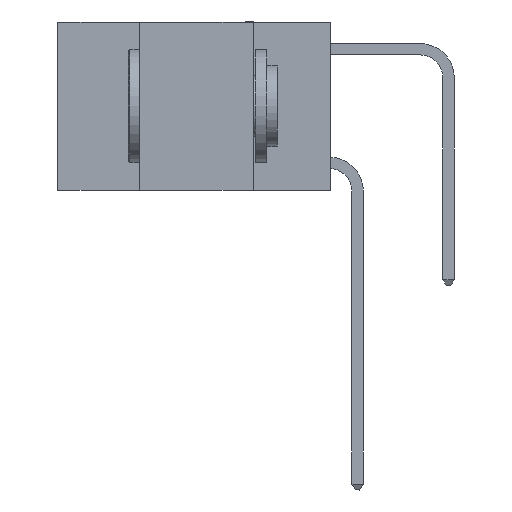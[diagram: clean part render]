
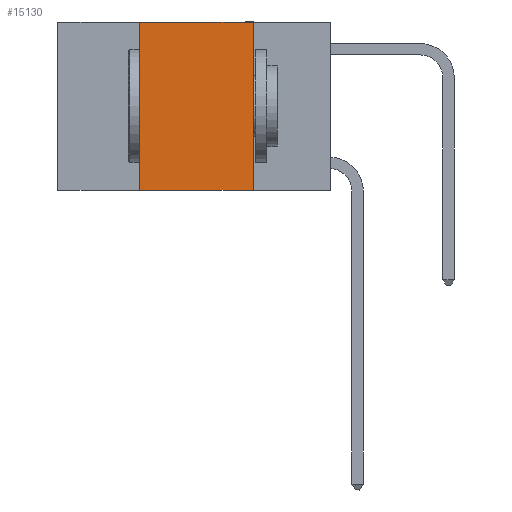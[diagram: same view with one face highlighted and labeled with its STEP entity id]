
A CAD part, left-side view. The second image highlights one B-rep face of the part: STEP entity #15130.
In plain terms, the highlighted planar face has unit normal (-1, 0, 0).
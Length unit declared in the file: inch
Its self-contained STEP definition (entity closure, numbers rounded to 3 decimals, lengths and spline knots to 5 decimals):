
#599 = LINE ( 'NONE', #7512, #14820 ) ;
#1552 = CARTESIAN_POINT ( 'NONE',  ( 0., 0.6, 0. ) ) ;
#2569 = AXIS2_PLACEMENT_3D ( 'NONE', #1552, #24740, #5537 ) ;
#2822 = EDGE_CURVE ( 'NONE', #22975, #13338, #5802, .T. ) ;
#3178 = ORIENTED_EDGE ( 'NONE', *, *, #8623, .F. ) ;
#3203 = ORIENTED_EDGE ( 'NONE', *, *, #2822, .T. ) ;
#3492 = PLANE ( 'NONE',  #2569 ) ;
#4155 = CARTESIAN_POINT ( 'NONE',  ( 0., 0.17, -0.37 ) ) ;
#4890 = DIRECTION ( 'NONE',  ( 0., 0., 1. ) ) ;
#5073 = DIRECTION ( 'NONE',  ( 0., -1., 0. ) ) ;
#5537 = DIRECTION ( 'NONE',  ( 0., 0., -1. ) ) ;
#5802 = LINE ( 'NONE', #12275, #10762 ) ;
#7512 = CARTESIAN_POINT ( 'NONE',  ( 0., 0.17, 0. ) ) ;
#8623 = EDGE_CURVE ( 'NONE', #11925, #20323, #9835, .T. ) ;
#8648 = EDGE_LOOP ( 'NONE', ( #23284, #3178, #22267, #3203 ) ) ;
#9672 = FACE_OUTER_BOUND ( 'NONE', #8648, .T. ) ;
#9835 = LINE ( 'NONE', #24299, #11509 ) ;
#10762 = VECTOR ( 'NONE', #17153, 39.37008 ) ;
#11509 = VECTOR ( 'NONE', #5073, 39.37008 ) ;
#11634 = CARTESIAN_POINT ( 'NONE',  ( 0., 0.42, 0. ) ) ;
#11925 = VERTEX_POINT ( 'NONE', #18303 ) ;
#12275 = CARTESIAN_POINT ( 'NONE',  ( 0., 0.6, -0.37 ) ) ;
#12483 = EDGE_CURVE ( 'NONE', #20323, #13338, #599, .T. ) ;
#13338 = VERTEX_POINT ( 'NONE', #4155 ) ;
#14820 = VECTOR ( 'NONE', #26689, 39.37008 ) ;
#15094 = EDGE_CURVE ( 'NONE', #22975, #11925, #22338, .T. ) ;
#15130 = ADVANCED_FACE ( 'NONE', ( #9672 ), #3492, .F. ) ;
#16221 = CARTESIAN_POINT ( 'NONE',  ( 0., 0.17, 0. ) ) ;
#17153 = DIRECTION ( 'NONE',  ( 0., -1., 0. ) ) ;
#18303 = CARTESIAN_POINT ( 'NONE',  ( 0., 0.42, 0. ) ) ;
#20323 = VERTEX_POINT ( 'NONE', #16221 ) ;
#22267 = ORIENTED_EDGE ( 'NONE', *, *, #15094, .F. ) ;
#22338 = LINE ( 'NONE', #11634, #26613 ) ;
#22975 = VERTEX_POINT ( 'NONE', #23719 ) ;
#23284 = ORIENTED_EDGE ( 'NONE', *, *, #12483, .F. ) ;
#23719 = CARTESIAN_POINT ( 'NONE',  ( 0., 0.42, -0.37 ) ) ;
#24299 = CARTESIAN_POINT ( 'NONE',  ( 0., 0.6, 0. ) ) ;
#24740 = DIRECTION ( 'NONE',  ( 1., 0., 0. ) ) ;
#26613 = VECTOR ( 'NONE', #4890, 39.37008 ) ;
#26689 = DIRECTION ( 'NONE',  ( 0., 0., -1. ) ) ;
